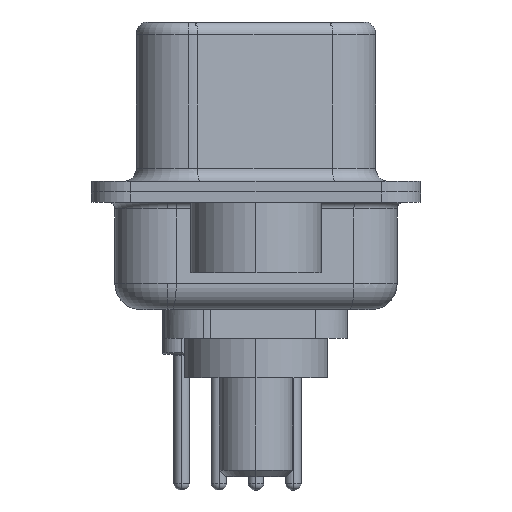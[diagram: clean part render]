
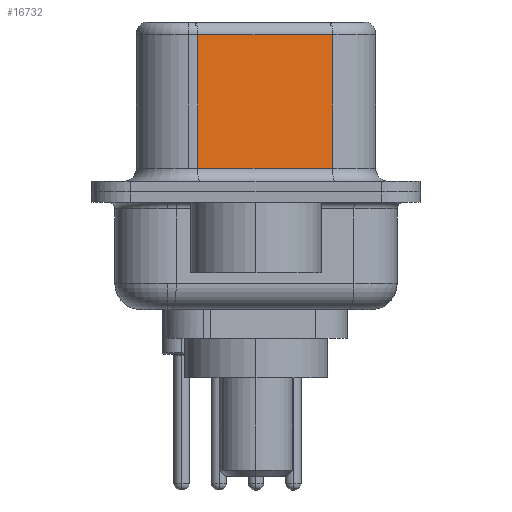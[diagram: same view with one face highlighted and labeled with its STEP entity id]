
A CAD part, left-side view. The second image highlights one B-rep face of the part: STEP entity #16732.
In plain terms, the highlighted planar face has unit normal (-0.985, -0.174, 0).
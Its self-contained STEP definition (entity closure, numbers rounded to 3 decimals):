
#1037 = EDGE_CURVE ( 'NONE', #1984, #20168, #19938, .T. ) ;
#1144 = DIRECTION ( 'NONE',  ( 0., 0., -1. ) ) ;
#1984 = VERTEX_POINT ( 'NONE', #18384 ) ;
#2127 = VECTOR ( 'NONE', #1144, 1000. ) ;
#2189 = DIRECTION ( 'NONE',  ( -0.174, 0.985, 0. ) ) ;
#3012 = AXIS2_PLACEMENT_3D ( 'NONE', #9979, #11587, #2189 ) ;
#4227 = ORIENTED_EDGE ( 'NONE', *, *, #8111, .T. ) ;
#5823 = CARTESIAN_POINT ( 'NONE',  ( 3.67, 2.233, 0.9 ) ) ;
#6238 = LINE ( 'NONE', #12119, #2127 ) ;
#6678 = VECTOR ( 'NONE', #14086, 1000. ) ;
#7176 = VERTEX_POINT ( 'NONE', #13361 ) ;
#7322 = DIRECTION ( 'NONE',  ( -0.174, 0.985, 0. ) ) ;
#7397 = DIRECTION ( 'NONE',  ( 0., 0., -1. ) ) ;
#7494 = VECTOR ( 'NONE', #7322, 1000. ) ;
#7655 = LINE ( 'NONE', #12518, #6678 ) ;
#7746 = ORIENTED_EDGE ( 'NONE', *, *, #15108, .T. ) ;
#8111 = EDGE_CURVE ( 'NONE', #12320, #20168, #7655, .T. ) ;
#8480 = LINE ( 'NONE', #15179, #7494 ) ;
#8780 = ORIENTED_EDGE ( 'NONE', *, *, #1037, .F. ) ;
#9979 = CARTESIAN_POINT ( 'NONE',  ( 4.58, -2.927, 6.52 ) ) ;
#11188 = FACE_OUTER_BOUND ( 'NONE', #15359, .T. ) ;
#11587 = DIRECTION ( 'NONE',  ( 0.985, 0.174, 0. ) ) ;
#12119 = CARTESIAN_POINT ( 'NONE',  ( 3.67, 2.233, 6.52 ) ) ;
#12261 = EDGE_CURVE ( 'NONE', #1984, #7176, #8480, .T. ) ;
#12320 = VERTEX_POINT ( 'NONE', #5823 ) ;
#12431 = ORIENTED_EDGE ( 'NONE', *, *, #12261, .T. ) ;
#12518 = CARTESIAN_POINT ( 'NONE',  ( 4.58, -2.927, 0.9 ) ) ;
#13361 = CARTESIAN_POINT ( 'NONE',  ( 3.67, 2.233, 6.02 ) ) ;
#14086 = DIRECTION ( 'NONE',  ( 0.174, -0.985, 0. ) ) ;
#15108 = EDGE_CURVE ( 'NONE', #7176, #12320, #6238, .T. ) ;
#15179 = CARTESIAN_POINT ( 'NONE',  ( 4.58, -2.927, 6.02 ) ) ;
#15359 = EDGE_LOOP ( 'NONE', ( #8780, #12431, #7746, #4227 ) ) ;
#15794 = VECTOR ( 'NONE', #7397, 1000. ) ;
#16417 = CARTESIAN_POINT ( 'NONE',  ( 4.58, -2.927, 6.52 ) ) ;
#16732 = ADVANCED_FACE ( 'NONE', ( #11188 ), #19435, .F. ) ;
#18384 = CARTESIAN_POINT ( 'NONE',  ( 4.58, -2.927, 6.02 ) ) ;
#19285 = CARTESIAN_POINT ( 'NONE',  ( 4.58, -2.927, 0.9 ) ) ;
#19435 = PLANE ( 'NONE',  #3012 ) ;
#19938 = LINE ( 'NONE', #16417, #15794 ) ;
#20168 = VERTEX_POINT ( 'NONE', #19285 ) ;
